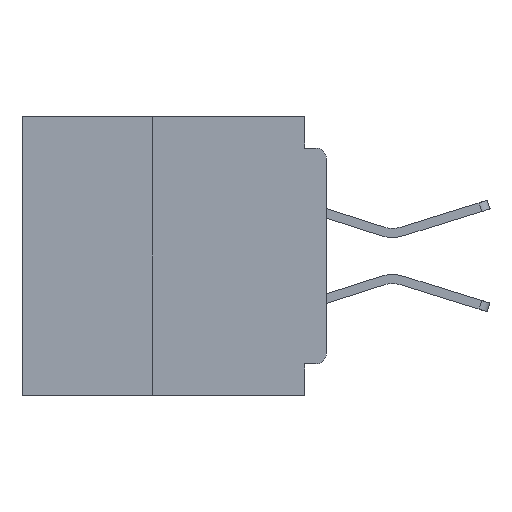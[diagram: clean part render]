
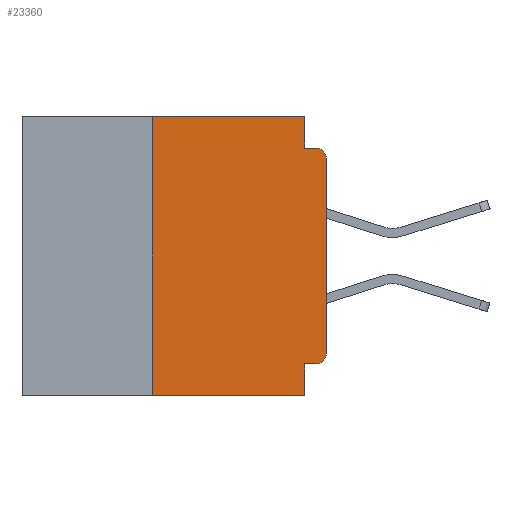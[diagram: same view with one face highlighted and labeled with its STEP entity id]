
A CAD part, left-side view. The second image highlights one B-rep face of the part: STEP entity #23360.
In plain terms, the highlighted planar face has unit normal (-1, 0, 0).
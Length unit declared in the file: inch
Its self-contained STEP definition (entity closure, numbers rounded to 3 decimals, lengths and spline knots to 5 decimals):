
#36 = DIRECTION ( 'NONE',  ( 0., 1., 0. ) ) ;
#324 = ORIENTED_EDGE ( 'NONE', *, *, #33164, .T. ) ;
#504 = DIRECTION ( 'NONE',  ( 0., 0., 1. ) ) ;
#714 = EDGE_CURVE ( 'NONE', #24868, #4457, #19636, .T. ) ;
#766 = ORIENTED_EDGE ( 'NONE', *, *, #28897, .T. ) ;
#1201 = DIRECTION ( 'NONE',  ( 0., -1., 0. ) ) ;
#1298 = DIRECTION ( 'NONE',  ( 0., 0., -1. ) ) ;
#2263 = CARTESIAN_POINT ( 'NONE',  ( 0., 0.25, -0.4 ) ) ;
#2505 = VERTEX_POINT ( 'NONE', #35343 ) ;
#2561 = EDGE_LOOP ( 'NONE', ( #324, #6654, #3976, #17646, #36249, #36488, #32443, #18354, #6259, #766 ) ) ;
#2730 = CIRCLE ( 'NONE', #14059, 0.015 ) ;
#3734 = EDGE_CURVE ( 'NONE', #26110, #6115, #40798, .T. ) ;
#3976 = ORIENTED_EDGE ( 'NONE', *, *, #3734, .F. ) ;
#4312 = CARTESIAN_POINT ( 'NONE',  ( 0., 0., -0.045 ) ) ;
#4457 = VERTEX_POINT ( 'NONE', #10954 ) ;
#4463 = LINE ( 'NONE', #25597, #11980 ) ;
#5796 = DIRECTION ( 'NONE',  ( 0., -1., 0. ) ) ;
#6115 = VERTEX_POINT ( 'NONE', #29334 ) ;
#6259 = ORIENTED_EDGE ( 'NONE', *, *, #33497, .F. ) ;
#6569 = LINE ( 'NONE', #37426, #22656 ) ;
#6654 = ORIENTED_EDGE ( 'NONE', *, *, #40164, .T. ) ;
#7796 = VERTEX_POINT ( 'NONE', #13280 ) ;
#7874 = EDGE_CURVE ( 'NONE', #39049, #26110, #16521, .T. ) ;
#8628 = DIRECTION ( 'NONE',  ( 0., -1., 0. ) ) ;
#9240 = VERTEX_POINT ( 'NONE', #14884 ) ;
#9867 = CARTESIAN_POINT ( 'NONE',  ( 0., 0.031, -0.045 ) ) ;
#10954 = CARTESIAN_POINT ( 'NONE',  ( 0., 0.25, 0. ) ) ;
#11074 = VECTOR ( 'NONE', #504, 39.37008 ) ;
#11087 = DIRECTION ( 'NONE',  ( 1., 0., 0. ) ) ;
#11980 = VECTOR ( 'NONE', #36, 39.37008 ) ;
#12452 = VERTEX_POINT ( 'NONE', #12987 ) ;
#12987 = CARTESIAN_POINT ( 'NONE',  ( 0., 0.031, -0.4 ) ) ;
#13280 = CARTESIAN_POINT ( 'NONE',  ( 0., 0., -0.34 ) ) ;
#14059 = AXIS2_PLACEMENT_3D ( 'NONE', #18321, #40533, #21530 ) ;
#14129 = VECTOR ( 'NONE', #5796, 39.37008 ) ;
#14884 = CARTESIAN_POINT ( 'NONE',  ( 0., 0.031, -0.355 ) ) ;
#15500 = VECTOR ( 'NONE', #20298, 39.37008 ) ;
#16182 = EDGE_CURVE ( 'NONE', #4457, #39049, #18682, .T. ) ;
#16336 = CARTESIAN_POINT ( 'NONE',  ( 0., 0.25, -0.4 ) ) ;
#16521 = LINE ( 'NONE', #23507, #15500 ) ;
#16590 = VECTOR ( 'NONE', #36558, 39.37008 ) ;
#17580 = LINE ( 'NONE', #39724, #16590 ) ;
#17646 = ORIENTED_EDGE ( 'NONE', *, *, #7874, .F. ) ;
#18136 = CARTESIAN_POINT ( 'NONE',  ( 0., 0.031, 0. ) ) ;
#18321 = CARTESIAN_POINT ( 'NONE',  ( 0., 0.015, -0.06 ) ) ;
#18354 = ORIENTED_EDGE ( 'NONE', *, *, #31447, .F. ) ;
#18371 = DIRECTION ( 'NONE',  ( 0., 0., -1. ) ) ;
#18682 = LINE ( 'NONE', #34109, #34601 ) ;
#19636 = LINE ( 'NONE', #2263, #11074 ) ;
#19927 = FACE_OUTER_BOUND ( 'NONE', #2561, .T. ) ;
#20298 = DIRECTION ( 'NONE',  ( 0., 0., -1. ) ) ;
#20552 = DIRECTION ( 'NONE',  ( -1., 0., 0. ) ) ;
#21530 = DIRECTION ( 'NONE',  ( 0., 0., -1. ) ) ;
#22656 = VECTOR ( 'NONE', #18371, 39.37008 ) ;
#23360 = ADVANCED_FACE ( 'NONE', ( #19927 ), #30280, .F. ) ;
#23507 = CARTESIAN_POINT ( 'NONE',  ( 0., 0.031, 0. ) ) ;
#23949 = VECTOR ( 'NONE', #1201, 39.37008 ) ;
#24868 = VERTEX_POINT ( 'NONE', #16336 ) ;
#24941 = CIRCLE ( 'NONE', #34434, 0.015 ) ;
#25597 = CARTESIAN_POINT ( 'NONE',  ( 0., 0., -0.355 ) ) ;
#26110 = VERTEX_POINT ( 'NONE', #9867 ) ;
#27056 = CARTESIAN_POINT ( 'NONE',  ( 0., 0.015, -0.355 ) ) ;
#28897 = EDGE_CURVE ( 'NONE', #31261, #7796, #24941, .T. ) ;
#29334 = CARTESIAN_POINT ( 'NONE',  ( 0., 0.015, -0.045 ) ) ;
#30280 = PLANE ( 'NONE',  #40365 ) ;
#31261 = VERTEX_POINT ( 'NONE', #27056 ) ;
#31280 = CARTESIAN_POINT ( 'NONE',  ( 0., 0.437, -0.4 ) ) ;
#31447 = EDGE_CURVE ( 'NONE', #9240, #12452, #6569, .T. ) ;
#32176 = EDGE_CURVE ( 'NONE', #24868, #12452, #38551, .T. ) ;
#32443 = ORIENTED_EDGE ( 'NONE', *, *, #32176, .T. ) ;
#33164 = EDGE_CURVE ( 'NONE', #7796, #2505, #17580, .T. ) ;
#33446 = DIRECTION ( 'NONE',  ( 0., 0., -1. ) ) ;
#33497 = EDGE_CURVE ( 'NONE', #31261, #9240, #4463, .T. ) ;
#34109 = CARTESIAN_POINT ( 'NONE',  ( 0., 0.437, 0. ) ) ;
#34434 = AXIS2_PLACEMENT_3D ( 'NONE', #39553, #20552, #1298 ) ;
#34601 = VECTOR ( 'NONE', #8628, 39.37008 ) ;
#35343 = CARTESIAN_POINT ( 'NONE',  ( 0., 0., -0.06 ) ) ;
#36249 = ORIENTED_EDGE ( 'NONE', *, *, #16182, .F. ) ;
#36488 = ORIENTED_EDGE ( 'NONE', *, *, #714, .F. ) ;
#36497 = CARTESIAN_POINT ( 'NONE',  ( 0., 0.437, 0. ) ) ;
#36558 = DIRECTION ( 'NONE',  ( 0., 0., 1. ) ) ;
#37426 = CARTESIAN_POINT ( 'NONE',  ( 0., 0.031, -0.4 ) ) ;
#38551 = LINE ( 'NONE', #31280, #14129 ) ;
#39049 = VERTEX_POINT ( 'NONE', #18136 ) ;
#39553 = CARTESIAN_POINT ( 'NONE',  ( 0., 0.015, -0.34 ) ) ;
#39724 = CARTESIAN_POINT ( 'NONE',  ( 0., 0., 0. ) ) ;
#40164 = EDGE_CURVE ( 'NONE', #2505, #6115, #2730, .T. ) ;
#40365 = AXIS2_PLACEMENT_3D ( 'NONE', #36497, #11087, #33446 ) ;
#40533 = DIRECTION ( 'NONE',  ( -1., 0., 0. ) ) ;
#40798 = LINE ( 'NONE', #4312, #23949 ) ;
